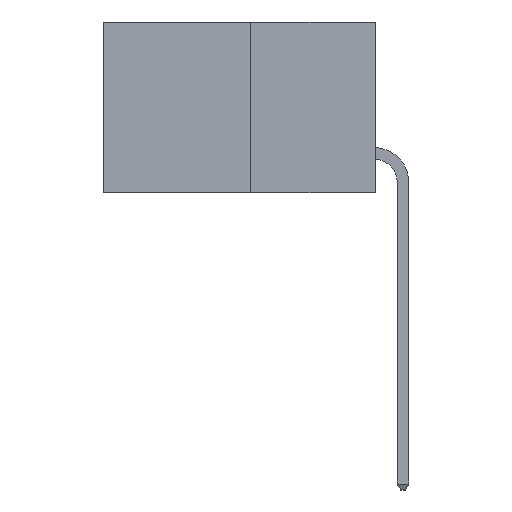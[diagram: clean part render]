
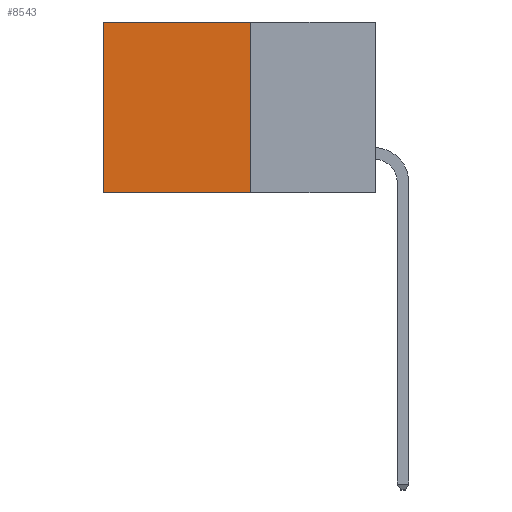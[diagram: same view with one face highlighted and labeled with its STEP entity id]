
A CAD part, left-side view. The second image highlights one B-rep face of the part: STEP entity #8543.
In plain terms, the highlighted planar face has unit normal (-1, 0, 0).
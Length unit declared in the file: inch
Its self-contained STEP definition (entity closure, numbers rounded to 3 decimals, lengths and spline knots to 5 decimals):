
#690 = VECTOR ( 'NONE', #12384, 39.37008 ) ;
#2763 = EDGE_LOOP ( 'NONE', ( #14979, #17144, #12690, #3654 ) ) ;
#3654 = ORIENTED_EDGE ( 'NONE', *, *, #15305, .T. ) ;
#4064 = CARTESIAN_POINT ( 'NONE',  ( 0.277, 0.59, -0.37 ) ) ;
#4297 = LINE ( 'NONE', #15881, #12598 ) ;
#4566 = DIRECTION ( 'NONE',  ( 0., 0., -1. ) ) ;
#4733 = VERTEX_POINT ( 'NONE', #7712 ) ;
#5178 = EDGE_CURVE ( 'NONE', #19680, #4733, #5635, .T. ) ;
#5438 = EDGE_CURVE ( 'NONE', #11009, #13951, #4297, .T. ) ;
#5635 = LINE ( 'NONE', #4064, #9520 ) ;
#5767 = PLANE ( 'NONE',  #13009 ) ;
#6503 = EDGE_CURVE ( 'NONE', #13951, #4733, #18004, .T. ) ;
#6957 = CARTESIAN_POINT ( 'NONE',  ( 0.277, 0.27, -0.37 ) ) ;
#7432 = DIRECTION ( 'NONE',  ( 1., 0., 0. ) ) ;
#7712 = CARTESIAN_POINT ( 'NONE',  ( 0.277, 0.59, -0.37 ) ) ;
#7852 = FACE_OUTER_BOUND ( 'NONE', #2763, .T. ) ;
#8543 = ADVANCED_FACE ( 'NONE', ( #7852 ), #5767, .F. ) ;
#8614 = CARTESIAN_POINT ( 'NONE',  ( 0.277, 0.59, 0. ) ) ;
#9239 = VECTOR ( 'NONE', #13820, 39.37008 ) ;
#9520 = VECTOR ( 'NONE', #4566, 39.37008 ) ;
#10106 = LINE ( 'NONE', #12308, #690 ) ;
#11009 = VERTEX_POINT ( 'NONE', #19637 ) ;
#12154 = CARTESIAN_POINT ( 'NONE',  ( 0.277, 0.27, -0.37 ) ) ;
#12308 = CARTESIAN_POINT ( 'NONE',  ( 0.277, 0.27, 0. ) ) ;
#12384 = DIRECTION ( 'NONE',  ( 0., 1., 0. ) ) ;
#12598 = VECTOR ( 'NONE', #15650, 39.37008 ) ;
#12690 = ORIENTED_EDGE ( 'NONE', *, *, #5438, .F. ) ;
#13009 = AXIS2_PLACEMENT_3D ( 'NONE', #17297, #7432, #18936 ) ;
#13820 = DIRECTION ( 'NONE',  ( 0., 1., 0. ) ) ;
#13951 = VERTEX_POINT ( 'NONE', #6957 ) ;
#14979 = ORIENTED_EDGE ( 'NONE', *, *, #5178, .T. ) ;
#15305 = EDGE_CURVE ( 'NONE', #11009, #19680, #10106, .T. ) ;
#15650 = DIRECTION ( 'NONE',  ( 0., 0., -1. ) ) ;
#15881 = CARTESIAN_POINT ( 'NONE',  ( 0.277, 0.27, -0.37 ) ) ;
#17144 = ORIENTED_EDGE ( 'NONE', *, *, #6503, .F. ) ;
#17297 = CARTESIAN_POINT ( 'NONE',  ( 0.277, 0.27, -0.37 ) ) ;
#18004 = LINE ( 'NONE', #12154, #9239 ) ;
#18936 = DIRECTION ( 'NONE',  ( 0., 0., -1. ) ) ;
#19637 = CARTESIAN_POINT ( 'NONE',  ( 0.277, 0.27, 0. ) ) ;
#19680 = VERTEX_POINT ( 'NONE', #8614 ) ;
